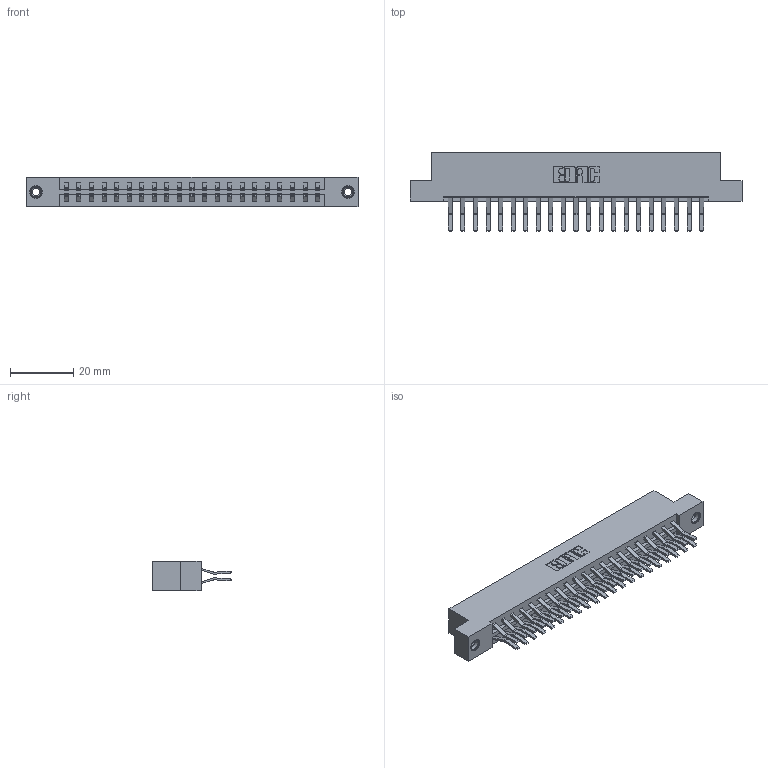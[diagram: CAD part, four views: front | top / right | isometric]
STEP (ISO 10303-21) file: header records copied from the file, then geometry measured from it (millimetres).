
FILE_DESCRIPTION (( 'STEP AP203' ), '1' );
FILE_NAME ('833-042-560-208.STEP', '2020-06-03T22:59:27', ( '' ), ( '' ), 'SwSTEP 2.0', 'SolidWorks 2020', '' );
FILE_SCHEMA (( 'CONFIG_CONTROL_DESIGN' ));
Length unit declared in the file: inch
Products named in the file (4): 345-292-001_560 Tail; 833 Part_Flush - .156 Dia - TI; 833-042-560-208; 345-250-001_345-250-003-102
Assembly tree (45 placements, depth 2):
  833-042-560-208
    833 Part_Flush - .156 Dia - TI
    345-292-001_560 Tail  x42
    345-250-001_345-250-003-102  x2
Bounding box: 104.75 x 24.78 x 9.4 mm (x, y, z)
Volume: 10766.7 mm3; surface area: 13310.4 mm2
Topology: 45 solids, 45 shells, 2442 faces, 7209 edges, 4742 vertices
Faces by surface type: plane 1614, cylinder 812, cone 12, torus 4
Entity records: 17500 total; most frequent: CARTESIAN_POINT 2909, ORIENTED_EDGE 2838, DIRECTION 2557, EDGE_CURVE 1419, LINE 1267, VECTOR 1267, VERTEX_POINT 940, AXIS2_PLACEMENT_3D 645
